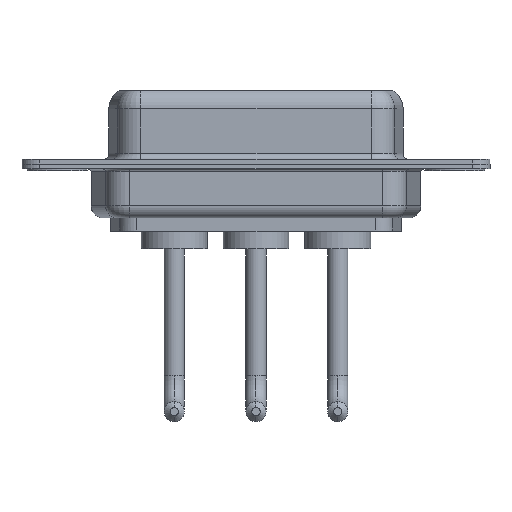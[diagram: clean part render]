
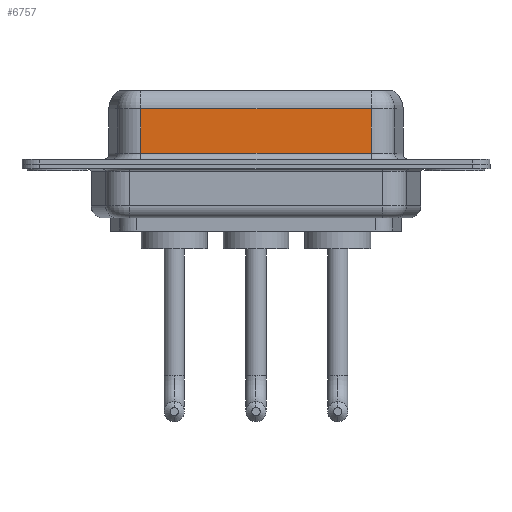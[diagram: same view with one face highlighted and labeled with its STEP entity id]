
A CAD part, front view. The second image highlights one B-rep face of the part: STEP entity #6757.
In plain terms, the highlighted planar face has unit normal (0, -1, 0).
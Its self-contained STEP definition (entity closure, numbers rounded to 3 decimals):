
#197 = DIRECTION ( 'NONE',  ( 1., 0., 0. ) ) ;
#395 = FACE_OUTER_BOUND ( 'NONE', #1226, .T. ) ;
#865 = CARTESIAN_POINT ( 'NONE',  ( 7.013, -3.95, 6.4 ) ) ;
#1151 = VECTOR ( 'NONE', #197, 1000. ) ;
#1195 = VECTOR ( 'NONE', #8022, 1000. ) ;
#1215 = ORIENTED_EDGE ( 'NONE', *, *, #7124, .T. ) ;
#1226 = EDGE_LOOP ( 'NONE', ( #8017, #4097, #1215, #5707 ) ) ;
#1289 = EDGE_CURVE ( 'NONE', #4952, #9562, #4135, .T. ) ;
#1558 = AXIS2_PLACEMENT_3D ( 'NONE', #5993, #8318, #2712 ) ;
#2486 = CARTESIAN_POINT ( 'NONE',  ( 26.287, -3.95, 6.4 ) ) ;
#2712 = DIRECTION ( 'NONE',  ( 0., 0., 1. ) ) ;
#2942 = CARTESIAN_POINT ( 'NONE',  ( 26.287, -3.95, 0.9 ) ) ;
#3163 = VECTOR ( 'NONE', #3974, 1000. ) ;
#3933 = CARTESIAN_POINT ( 'NONE',  ( 26.287, -3.95, 4.65 ) ) ;
#3974 = DIRECTION ( 'NONE',  ( 0., 0., -1. ) ) ;
#4097 = ORIENTED_EDGE ( 'NONE', *, *, #6078, .T. ) ;
#4135 = LINE ( 'NONE', #2486, #3163 ) ;
#4136 = DIRECTION ( 'NONE',  ( 0., 0., -1. ) ) ;
#4952 = VERTEX_POINT ( 'NONE', #3933 ) ;
#5128 = VECTOR ( 'NONE', #4136, 1000. ) ;
#5707 = ORIENTED_EDGE ( 'NONE', *, *, #9501, .T. ) ;
#5714 = CARTESIAN_POINT ( 'NONE',  ( 7.013, -3.95, 0.9 ) ) ;
#5746 = VERTEX_POINT ( 'NONE', #6451 ) ;
#5993 = CARTESIAN_POINT ( 'NONE',  ( 26.287, -3.95, 6.4 ) ) ;
#6078 = EDGE_CURVE ( 'NONE', #4952, #5746, #8713, .T. ) ;
#6451 = CARTESIAN_POINT ( 'NONE',  ( 7.013, -3.95, 4.65 ) ) ;
#6655 = LINE ( 'NONE', #7503, #1151 ) ;
#6757 = ADVANCED_FACE ( 'NONE', ( #395 ), #9067, .F. ) ;
#7124 = EDGE_CURVE ( 'NONE', #5746, #9969, #8146, .T. ) ;
#7503 = CARTESIAN_POINT ( 'NONE',  ( 26.287, -3.95, 0.9 ) ) ;
#8017 = ORIENTED_EDGE ( 'NONE', *, *, #1289, .F. ) ;
#8022 = DIRECTION ( 'NONE',  ( -1., 0., 0. ) ) ;
#8146 = LINE ( 'NONE', #865, #5128 ) ;
#8318 = DIRECTION ( 'NONE',  ( 0., 1., 0. ) ) ;
#8713 = LINE ( 'NONE', #9518, #1195 ) ;
#9067 = PLANE ( 'NONE',  #1558 ) ;
#9501 = EDGE_CURVE ( 'NONE', #9969, #9562, #6655, .T. ) ;
#9518 = CARTESIAN_POINT ( 'NONE',  ( 26.287, -3.95, 4.65 ) ) ;
#9562 = VERTEX_POINT ( 'NONE', #2942 ) ;
#9969 = VERTEX_POINT ( 'NONE', #5714 ) ;
